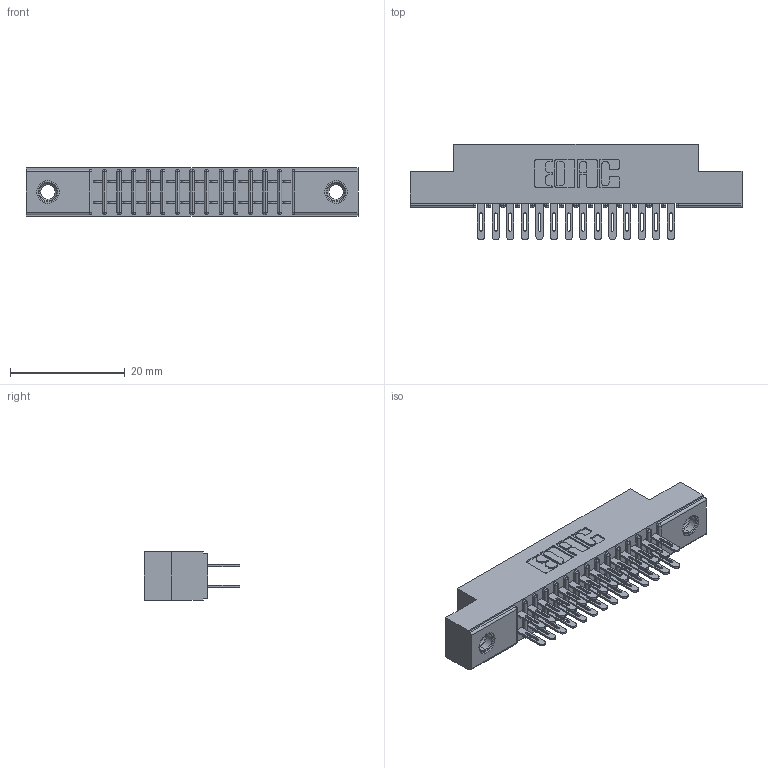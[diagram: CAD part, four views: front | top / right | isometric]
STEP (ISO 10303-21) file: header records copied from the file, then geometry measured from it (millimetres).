
FILE_DESCRIPTION (( 'STEP AP203' ), '1' );
FILE_NAME ('341-028-500-207.STEP', '2018-08-06T19:12:45', ( '' ), ( '' ), 'SwSTEP 2.0', 'SolidWorks 2016', '' );
FILE_SCHEMA (( 'CONFIG_CONTROL_DESIGN' ));
Length unit declared in the file: inch
Products named in the file (4): 341-292-001_341-292-100; 345-250-001_345-250-005-103; 341-028-500-207; 341 Part_.156 (3.96) Dia Mounting Holes
Assembly tree (31 placements, depth 2):
  341-028-500-207
    341 Part_.156 (3.96) Dia Mounting Holes
    341-292-001_341-292-100  x28
    345-250-001_345-250-005-103  x2
Bounding box: 57.78 x 16.69 x 8.38 mm (x, y, z)
Volume: 3334.2 mm3; surface area: 6713.6 mm2
Topology: 31 solids, 31 shells, 2024 faces, 5814 edges, 3762 vertices
Faces by surface type: plane 1164, cylinder 788, sphere 30, torus 30, cone 12
Entity records: 21866 total; most frequent: CARTESIAN_POINT 3617, ORIENTED_EDGE 3584, DIRECTION 3544, EDGE_CURVE 1792, VECTOR 1410, LINE 1410, VERTEX_POINT 1140, AXIS2_PLACEMENT_3D 1067
